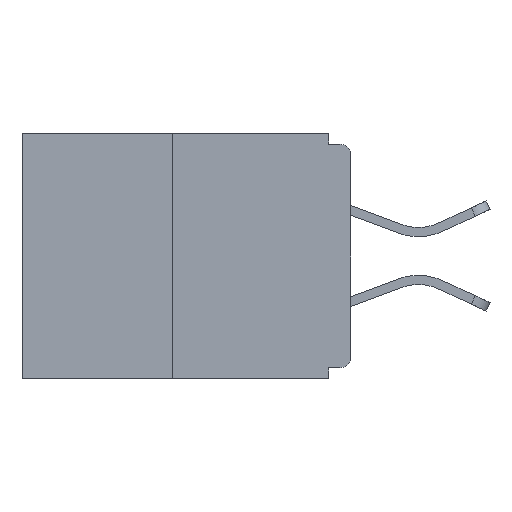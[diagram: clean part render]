
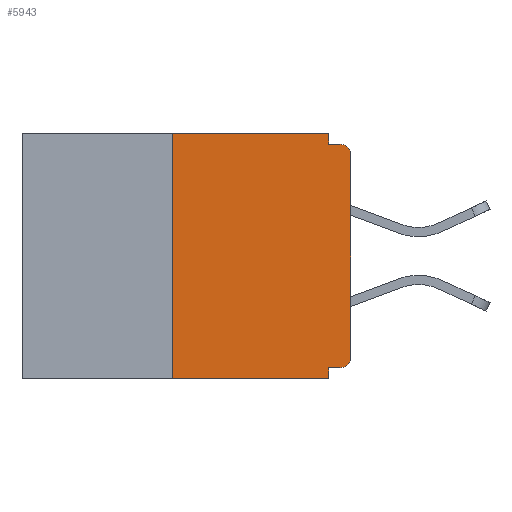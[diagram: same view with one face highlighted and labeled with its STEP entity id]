
A CAD part, left-side view. The second image highlights one B-rep face of the part: STEP entity #5943.
In plain terms, the highlighted planar face has unit normal (-1, 0, 0).
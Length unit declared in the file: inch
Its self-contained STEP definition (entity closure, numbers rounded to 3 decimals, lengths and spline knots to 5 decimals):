
#107 = LINE ( 'NONE', #10431, #11786 ) ;
#261 = VERTEX_POINT ( 'NONE', #12784 ) ;
#519 = VECTOR ( 'NONE', #4921, 39.37008 ) ;
#693 = ORIENTED_EDGE ( 'NONE', *, *, #3559, .T. ) ;
#729 = LINE ( 'NONE', #13673, #519 ) ;
#948 = EDGE_CURVE ( 'NONE', #10309, #261, #3909, .T. ) ;
#1193 = DIRECTION ( 'NONE',  ( 0., 0., 1. ) ) ;
#1422 = CARTESIAN_POINT ( 'NONE',  ( 0., 0.015, -0.015 ) ) ;
#2052 = EDGE_CURVE ( 'NONE', #8698, #11766, #13949, .T. ) ;
#2331 = LINE ( 'NONE', #13061, #15171 ) ;
#2414 = AXIS2_PLACEMENT_3D ( 'NONE', #15403, #6628, #18363 ) ;
#2440 = VECTOR ( 'NONE', #16356, 39.37008 ) ;
#2619 = DIRECTION ( 'NONE',  ( 0., -1., 0. ) ) ;
#3196 = VERTEX_POINT ( 'NONE', #13234 ) ;
#3294 = VERTEX_POINT ( 'NONE', #16759 ) ;
#3316 = ORIENTED_EDGE ( 'NONE', *, *, #14190, .T. ) ;
#3382 = ORIENTED_EDGE ( 'NONE', *, *, #6240, .F. ) ;
#3559 = EDGE_CURVE ( 'NONE', #11766, #13199, #6826, .T. ) ;
#3769 = DIRECTION ( 'NONE',  ( 1., 0., 0. ) ) ;
#3909 = LINE ( 'NONE', #15627, #12840 ) ;
#4223 = CARTESIAN_POINT ( 'NONE',  ( 0., 0.25, 0. ) ) ;
#4487 = CARTESIAN_POINT ( 'NONE',  ( 0., 0.25, 0. ) ) ;
#4684 = EDGE_CURVE ( 'NONE', #8698, #10309, #107, .T. ) ;
#4921 = DIRECTION ( 'NONE',  ( 0., -1., 0. ) ) ;
#5453 = EDGE_CURVE ( 'NONE', #3196, #16338, #729, .T. ) ;
#5943 = ADVANCED_FACE ( 'NONE', ( #18197 ), #10948, .F. ) ;
#6043 = DIRECTION ( 'NONE',  ( 0., 1., 0. ) ) ;
#6240 = EDGE_CURVE ( 'NONE', #13042, #6859, #8750, .T. ) ;
#6628 = DIRECTION ( 'NONE',  ( -1., 0., 0. ) ) ;
#6826 = LINE ( 'NONE', #8774, #2440 ) ;
#6859 = VERTEX_POINT ( 'NONE', #4487 ) ;
#7397 = DIRECTION ( 'NONE',  ( -1., 0., 0. ) ) ;
#8069 = ORIENTED_EDGE ( 'NONE', *, *, #2052, .T. ) ;
#8088 = AXIS2_PLACEMENT_3D ( 'NONE', #12414, #3769, #12480 ) ;
#8294 = VECTOR ( 'NONE', #8964, 39.37008 ) ;
#8531 = CARTESIAN_POINT ( 'NONE',  ( 0., 0., -0.313 ) ) ;
#8631 = ORIENTED_EDGE ( 'NONE', *, *, #5453, .F. ) ;
#8698 = VERTEX_POINT ( 'NONE', #16689 ) ;
#8750 = LINE ( 'NONE', #4223, #11953 ) ;
#8774 = CARTESIAN_POINT ( 'NONE',  ( 0., 0., 0. ) ) ;
#8964 = DIRECTION ( 'NONE',  ( 0., -1., 0. ) ) ;
#9418 = LINE ( 'NONE', #18016, #8294 ) ;
#10185 = DIRECTION ( 'NONE',  ( 0., 0., -1. ) ) ;
#10272 = ORIENTED_EDGE ( 'NONE', *, *, #11735, .T. ) ;
#10309 = VERTEX_POINT ( 'NONE', #11622 ) ;
#10358 = CIRCLE ( 'NONE', #2414, 0.015 ) ;
#10431 = CARTESIAN_POINT ( 'NONE',  ( 0., 0., -0.328 ) ) ;
#10578 = ORIENTED_EDGE ( 'NONE', *, *, #4684, .F. ) ;
#10653 = EDGE_LOOP ( 'NONE', ( #13979, #3382, #10272, #11079, #10578, #8069, #693, #3316, #8631, #15379 ) ) ;
#10675 = LINE ( 'NONE', #17158, #18978 ) ;
#10948 = PLANE ( 'NONE',  #8088 ) ;
#11079 = ORIENTED_EDGE ( 'NONE', *, *, #948, .F. ) ;
#11622 = CARTESIAN_POINT ( 'NONE',  ( 0., 0.031, -0.328 ) ) ;
#11735 = EDGE_CURVE ( 'NONE', #13042, #261, #10675, .T. ) ;
#11766 = VERTEX_POINT ( 'NONE', #8531 ) ;
#11786 = VECTOR ( 'NONE', #6043, 39.37008 ) ;
#11953 = VECTOR ( 'NONE', #1193, 39.37008 ) ;
#12098 = AXIS2_PLACEMENT_3D ( 'NONE', #16071, #7397, #16129 ) ;
#12414 = CARTESIAN_POINT ( 'NONE',  ( 0., 0.46, 0. ) ) ;
#12480 = DIRECTION ( 'NONE',  ( 0., 0., -1. ) ) ;
#12784 = CARTESIAN_POINT ( 'NONE',  ( 0., 0.031, -0.343 ) ) ;
#12840 = VECTOR ( 'NONE', #13985, 39.37008 ) ;
#13042 = VERTEX_POINT ( 'NONE', #17293 ) ;
#13061 = CARTESIAN_POINT ( 'NONE',  ( 0., 0.031, 0. ) ) ;
#13199 = VERTEX_POINT ( 'NONE', #18953 ) ;
#13234 = CARTESIAN_POINT ( 'NONE',  ( 0., 0.031, -0.015 ) ) ;
#13673 = CARTESIAN_POINT ( 'NONE',  ( 0., 0., -0.015 ) ) ;
#13949 = CIRCLE ( 'NONE', #12098, 0.015 ) ;
#13979 = ORIENTED_EDGE ( 'NONE', *, *, #14422, .F. ) ;
#13985 = DIRECTION ( 'NONE',  ( 0., 0., -1. ) ) ;
#14190 = EDGE_CURVE ( 'NONE', #13199, #16338, #10358, .T. ) ;
#14394 = EDGE_CURVE ( 'NONE', #3294, #3196, #2331, .T. ) ;
#14422 = EDGE_CURVE ( 'NONE', #6859, #3294, #9418, .T. ) ;
#15171 = VECTOR ( 'NONE', #10185, 39.37008 ) ;
#15379 = ORIENTED_EDGE ( 'NONE', *, *, #14394, .F. ) ;
#15403 = CARTESIAN_POINT ( 'NONE',  ( 0., 0.015, -0.03 ) ) ;
#15627 = CARTESIAN_POINT ( 'NONE',  ( 0., 0.031, -0.343 ) ) ;
#16071 = CARTESIAN_POINT ( 'NONE',  ( 0., 0.015, -0.313 ) ) ;
#16129 = DIRECTION ( 'NONE',  ( 0., 0., -1. ) ) ;
#16338 = VERTEX_POINT ( 'NONE', #1422 ) ;
#16356 = DIRECTION ( 'NONE',  ( 0., 0., 1. ) ) ;
#16689 = CARTESIAN_POINT ( 'NONE',  ( 0., 0.015, -0.328 ) ) ;
#16759 = CARTESIAN_POINT ( 'NONE',  ( 0., 0.031, 0. ) ) ;
#17158 = CARTESIAN_POINT ( 'NONE',  ( 0., 0.46, -0.343 ) ) ;
#17293 = CARTESIAN_POINT ( 'NONE',  ( 0., 0.25, -0.343 ) ) ;
#18016 = CARTESIAN_POINT ( 'NONE',  ( 0., 0.46, 0. ) ) ;
#18197 = FACE_OUTER_BOUND ( 'NONE', #10653, .T. ) ;
#18363 = DIRECTION ( 'NONE',  ( 0., 0., -1. ) ) ;
#18953 = CARTESIAN_POINT ( 'NONE',  ( 0., 0., -0.03 ) ) ;
#18978 = VECTOR ( 'NONE', #2619, 39.37008 ) ;
